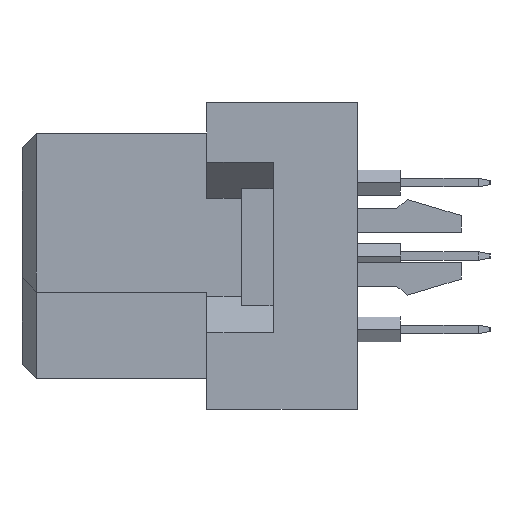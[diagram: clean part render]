
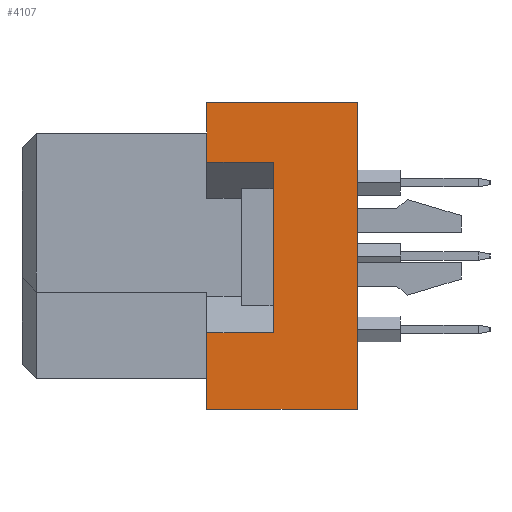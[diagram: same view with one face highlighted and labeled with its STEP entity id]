
A CAD part, left-side view. The second image highlights one B-rep face of the part: STEP entity #4107.
In plain terms, the highlighted planar face has unit normal (-1, 0, 0).
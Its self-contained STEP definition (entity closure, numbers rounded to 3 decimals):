
#397 = CARTESIAN_POINT ( 'NONE',  ( -47.5, -6.4, 3.25 ) ) ;
#1491 = CARTESIAN_POINT ( 'NONE',  ( -47.5, -6.4, -5.3 ) ) ;
#1569 = DIRECTION ( 'NONE',  ( 0., 1., 0. ) ) ;
#2161 = VERTEX_POINT ( 'NONE', #4308 ) ;
#2543 = DIRECTION ( 'NONE',  ( 0., 0., 1. ) ) ;
#2657 = ORIENTED_EDGE ( 'NONE', *, *, #33643, .F. ) ;
#2995 = DIRECTION ( 'NONE',  ( 0., 0., 1. ) ) ;
#3175 = LINE ( 'NONE', #25992, #5347 ) ;
#4107 = ADVANCED_FACE ( 'NONE', ( #5499 ), #5085, .T. ) ;
#4257 = VERTEX_POINT ( 'NONE', #16041 ) ;
#4261 = CARTESIAN_POINT ( 'NONE',  ( -47.5, -6.4, -5.3 ) ) ;
#4308 = CARTESIAN_POINT ( 'NONE',  ( -47.5, -6.4, -2.65 ) ) ;
#4492 = EDGE_LOOP ( 'NONE', ( #7294, #9077, #4946, #10288, #40119, #19647, #23213, #2657 ) ) ;
#4946 = ORIENTED_EDGE ( 'NONE', *, *, #31926, .F. ) ;
#5085 = PLANE ( 'NONE',  #23347 ) ;
#5347 = VECTOR ( 'NONE', #6544, 1000. ) ;
#5499 = FACE_OUTER_BOUND ( 'NONE', #4492, .T. ) ;
#5832 = EDGE_CURVE ( 'NONE', #8904, #2161, #33669, .T. ) ;
#6544 = DIRECTION ( 'NONE',  ( 0., 1., 0. ) ) ;
#7294 = ORIENTED_EDGE ( 'NONE', *, *, #5832, .T. ) ;
#7732 = LINE ( 'NONE', #24398, #10783 ) ;
#8072 = LINE ( 'NONE', #20954, #8576 ) ;
#8576 = VECTOR ( 'NONE', #33835, 1000. ) ;
#8904 = VERTEX_POINT ( 'NONE', #14083 ) ;
#9077 = ORIENTED_EDGE ( 'NONE', *, *, #28207, .F. ) ;
#9119 = LINE ( 'NONE', #35090, #28899 ) ;
#9450 = EDGE_CURVE ( 'NONE', #4257, #32920, #3175, .T. ) ;
#10288 = ORIENTED_EDGE ( 'NONE', *, *, #14763, .T. ) ;
#10783 = VECTOR ( 'NONE', #18061, 1000. ) ;
#11062 = VERTEX_POINT ( 'NONE', #33986 ) ;
#12858 = VERTEX_POINT ( 'NONE', #397 ) ;
#14083 = CARTESIAN_POINT ( 'NONE',  ( -47.5, -8.7, -2.65 ) ) ;
#14763 = EDGE_CURVE ( 'NONE', #11062, #4257, #7732, .T. ) ;
#15049 = CARTESIAN_POINT ( 'NONE',  ( -47.5, -8.7, 3.25 ) ) ;
#16041 = CARTESIAN_POINT ( 'NONE',  ( -47.5, -11.6, 5.3 ) ) ;
#17457 = EDGE_CURVE ( 'NONE', #12858, #32920, #27061, .T. ) ;
#18061 = DIRECTION ( 'NONE',  ( 0., 0., 1. ) ) ;
#18505 = VERTEX_POINT ( 'NONE', #15049 ) ;
#19647 = ORIENTED_EDGE ( 'NONE', *, *, #17457, .F. ) ;
#20308 = DIRECTION ( 'NONE',  ( 0., 0., 1. ) ) ;
#20954 = CARTESIAN_POINT ( 'NONE',  ( -47.5, -11.6, -5.3 ) ) ;
#21000 = CARTESIAN_POINT ( 'NONE',  ( -47.5, -6.4, -5.3 ) ) ;
#21340 = LINE ( 'NONE', #1491, #34687 ) ;
#22386 = VERTEX_POINT ( 'NONE', #21000 ) ;
#23213 = ORIENTED_EDGE ( 'NONE', *, *, #35509, .F. ) ;
#23347 = AXIS2_PLACEMENT_3D ( 'NONE', #31264, #28112, #2543 ) ;
#24398 = CARTESIAN_POINT ( 'NONE',  ( -47.5, -11.6, 5.3 ) ) ;
#25330 = DIRECTION ( 'NONE',  ( 0., 0., 1. ) ) ;
#25992 = CARTESIAN_POINT ( 'NONE',  ( -47.5, -11.6, 5.3 ) ) ;
#27061 = LINE ( 'NONE', #4261, #30493 ) ;
#28112 = DIRECTION ( 'NONE',  ( -1., 0., 0. ) ) ;
#28207 = EDGE_CURVE ( 'NONE', #22386, #2161, #21340, .T. ) ;
#28899 = VECTOR ( 'NONE', #2995, 1000. ) ;
#30475 = VECTOR ( 'NONE', #1569, 1000. ) ;
#30493 = VECTOR ( 'NONE', #20308, 1000. ) ;
#31264 = CARTESIAN_POINT ( 'NONE',  ( -47.5, -11.6, 5.3 ) ) ;
#31614 = DIRECTION ( 'NONE',  ( 0., 1., 0. ) ) ;
#31823 = LINE ( 'NONE', #34376, #36326 ) ;
#31926 = EDGE_CURVE ( 'NONE', #11062, #22386, #8072, .T. ) ;
#32920 = VERTEX_POINT ( 'NONE', #38728 ) ;
#33056 = CARTESIAN_POINT ( 'NONE',  ( -47.5, -8.7, -2.65 ) ) ;
#33643 = EDGE_CURVE ( 'NONE', #8904, #18505, #9119, .T. ) ;
#33669 = LINE ( 'NONE', #33056, #30475 ) ;
#33835 = DIRECTION ( 'NONE',  ( 0., 1., 0. ) ) ;
#33986 = CARTESIAN_POINT ( 'NONE',  ( -47.5, -11.6, -5.3 ) ) ;
#34376 = CARTESIAN_POINT ( 'NONE',  ( -47.5, -8.7, 3.25 ) ) ;
#34687 = VECTOR ( 'NONE', #25330, 1000. ) ;
#35090 = CARTESIAN_POINT ( 'NONE',  ( -47.5, -8.7, -2.65 ) ) ;
#35509 = EDGE_CURVE ( 'NONE', #18505, #12858, #31823, .T. ) ;
#36326 = VECTOR ( 'NONE', #31614, 1000. ) ;
#38728 = CARTESIAN_POINT ( 'NONE',  ( -47.5, -6.4, 5.3 ) ) ;
#40119 = ORIENTED_EDGE ( 'NONE', *, *, #9450, .T. ) ;
